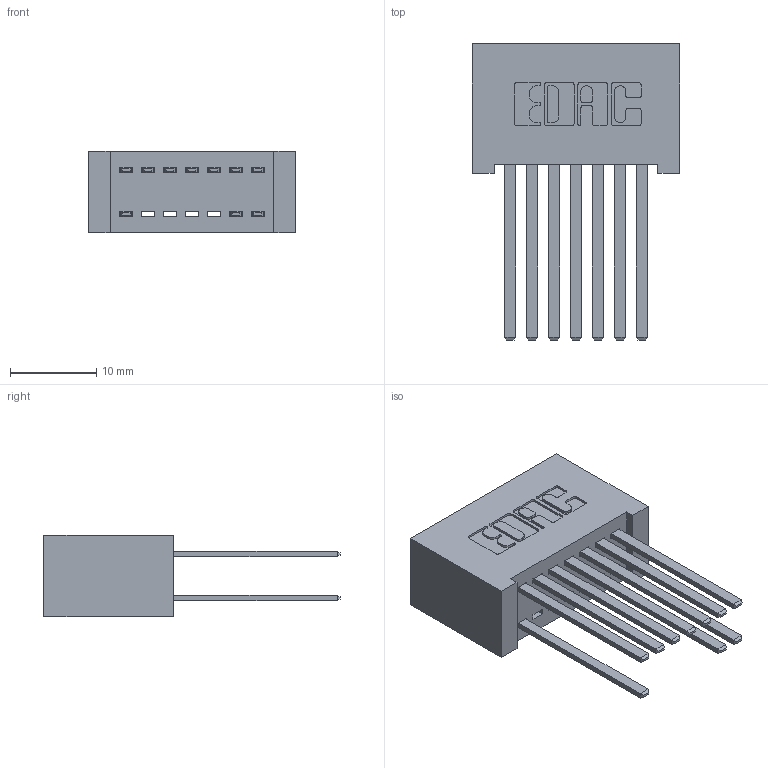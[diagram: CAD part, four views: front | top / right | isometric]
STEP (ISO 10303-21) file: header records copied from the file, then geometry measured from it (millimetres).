
FILE_DESCRIPTION (( 'STEP AP203' ), '1' );
FILE_NAME ('392-014-544-201.STEP', '2018-08-15T00:13:20', ( '' ), ( '' ), 'SwSTEP 2.0', 'SolidWorks 2016', '' );
FILE_SCHEMA (( 'CONFIG_CONTROL_DESIGN' ));
Length unit declared in the file: inch
Products named in the file (3): 342 Part_Lugless; 345-292-001_345-293-144; 392-014-544-201
Assembly tree (11 placements, depth 2):
  392-014-544-201
    342 Part_Lugless
    345-292-001_345-293-144  x10
Bounding box: 24.03 x 34.3 x 9.4 mm (x, y, z)
Volume: 2537 mm3; surface area: 3902.6 mm2
Topology: 11 solids, 11 shells, 586 faces, 1729 edges, 1138 vertices
Faces by surface type: plane 406, cylinder 180
Entity records: 8309 total; most frequent: CARTESIAN_POINT 1430, ORIENTED_EDGE 1370, DIRECTION 1269, EDGE_CURVE 685, LINE 569, VECTOR 569, VERTEX_POINT 454, AXIS2_PLACEMENT_3D 350
